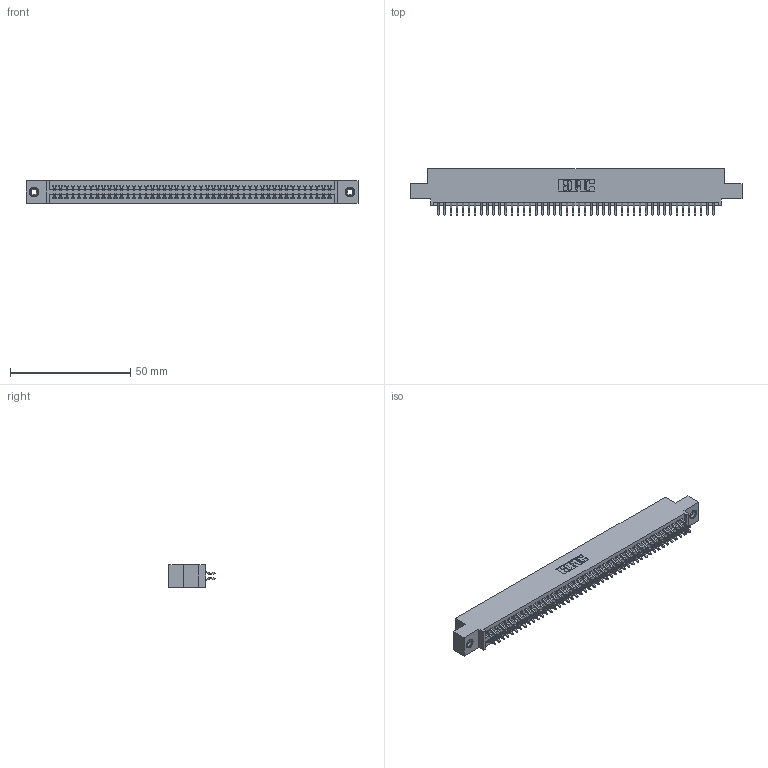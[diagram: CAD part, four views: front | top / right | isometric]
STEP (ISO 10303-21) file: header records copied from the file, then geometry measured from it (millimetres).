
FILE_DESCRIPTION (( 'STEP AP203' ), '1' );
FILE_NAME ('395-092-556-508.STEP', '2018-11-29T09:08:41', ( '' ), ( '' ), 'SwSTEP 2.0', 'SolidWorks 2016', '' );
FILE_SCHEMA (( 'CONFIG_CONTROL_DESIGN' ));
Length unit declared in the file: inch
Products named in the file (4): 345-292-001_556 Tail; 345 Part_0.110 Offset - 0.156 Dia-TI; 345-250-001_345-250-003-102; 395-092-556-508
Assembly tree (95 placements, depth 2):
  395-092-556-508
    345 Part_0.110 Offset - 0.156 Dia-TI
    345-292-001_556 Tail  x92
    345-250-001_345-250-003-102  x2
Bounding box: 138.05 x 19.24 x 9.4 mm (x, y, z)
Volume: 13363.8 mm3; surface area: 19857.2 mm2
Topology: 95 solids, 95 shells, 5342 faces, 15853 edges, 10438 vertices
Faces by surface type: plane 3520, cylinder 1806, cone 12, torus 4
Entity records: 37092 total; most frequent: CARTESIAN_POINT 6211, ORIENTED_EDGE 6126, DIRECTION 5485, EDGE_CURVE 3063, LINE 2719, VECTOR 2719, VERTEX_POINT 2036, AXIS2_PLACEMENT_3D 1383
